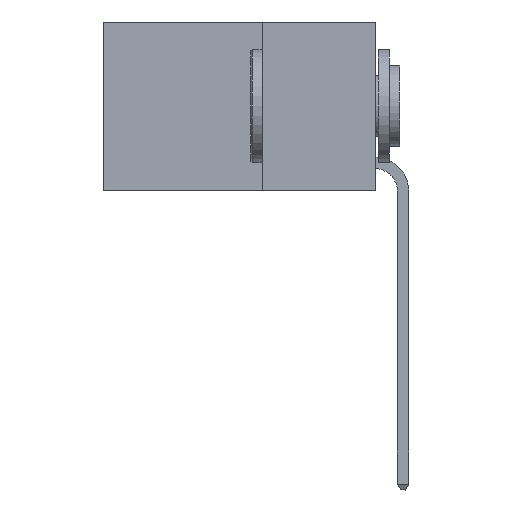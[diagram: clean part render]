
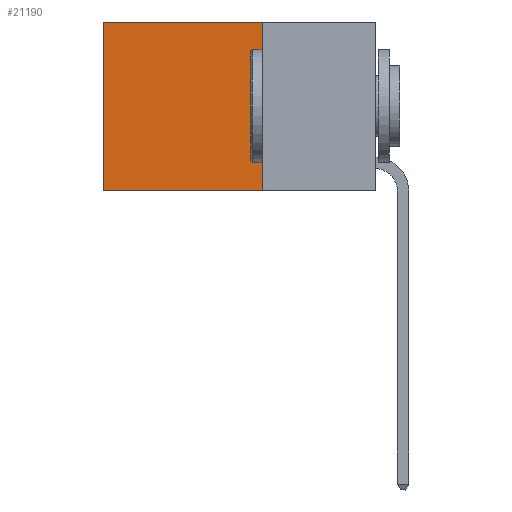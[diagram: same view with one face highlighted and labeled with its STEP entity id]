
A CAD part, left-side view. The second image highlights one B-rep face of the part: STEP entity #21190.
In plain terms, the highlighted planar face has unit normal (-1, 0, 0).
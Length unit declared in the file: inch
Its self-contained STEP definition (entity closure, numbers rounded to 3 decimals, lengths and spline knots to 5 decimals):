
#2144 = DIRECTION ( 'NONE',  ( 0., 1., 0. ) ) ;
#2157 = CARTESIAN_POINT ( 'NONE',  ( 0.2625, 0.25, 0. ) ) ;
#2172 = CARTESIAN_POINT ( 'NONE',  ( 0.2625, 0.6, 0. ) ) ;
#2182 = VECTOR ( 'NONE', #5967, 39.37008 ) ;
#2566 = CARTESIAN_POINT ( 'NONE',  ( 0.2625, 0.25, 0. ) ) ;
#3322 = VERTEX_POINT ( 'NONE', #19177 ) ;
#3429 = DIRECTION ( 'NONE',  ( 0., 0., -1. ) ) ;
#5967 = DIRECTION ( 'NONE',  ( 0., 1., 0. ) ) ;
#7459 = VERTEX_POINT ( 'NONE', #13827 ) ;
#7575 = CARTESIAN_POINT ( 'NONE',  ( 0.2625, 0.25, -0.37 ) ) ;
#7764 = ORIENTED_EDGE ( 'NONE', *, *, #11407, .T. ) ;
#7825 = LINE ( 'NONE', #2157, #2182 ) ;
#7829 = VECTOR ( 'NONE', #2144, 39.37008 ) ;
#9007 = EDGE_CURVE ( 'NONE', #7459, #3322, #13155, .T. ) ;
#11407 = EDGE_CURVE ( 'NONE', #19480, #3322, #18967, .T. ) ;
#11421 = LINE ( 'NONE', #16744, #15917 ) ;
#11435 = DIRECTION ( 'NONE',  ( 1., 0., 0. ) ) ;
#11440 = EDGE_LOOP ( 'NONE', ( #7764, #14529, #12044, #15341 ) ) ;
#11797 = EDGE_CURVE ( 'NONE', #14959, #19480, #7825, .T. ) ;
#12044 = ORIENTED_EDGE ( 'NONE', *, *, #20227, .F. ) ;
#13155 = LINE ( 'NONE', #7575, #7829 ) ;
#13446 = CARTESIAN_POINT ( 'NONE',  ( 0.2625, 0.25, 0. ) ) ;
#13447 = DIRECTION ( 'NONE',  ( 0., 0., -1. ) ) ;
#13827 = CARTESIAN_POINT ( 'NONE',  ( 0.2625, 0.25, -0.37 ) ) ;
#14010 = AXIS2_PLACEMENT_3D ( 'NONE', #2566, #11435, #22887 ) ;
#14529 = ORIENTED_EDGE ( 'NONE', *, *, #9007, .F. ) ;
#14959 = VERTEX_POINT ( 'NONE', #13446 ) ;
#15328 = PLANE ( 'NONE',  #14010 ) ;
#15341 = ORIENTED_EDGE ( 'NONE', *, *, #11797, .T. ) ;
#15696 = FACE_OUTER_BOUND ( 'NONE', #11440, .T. ) ;
#15917 = VECTOR ( 'NONE', #3429, 39.37008 ) ;
#16744 = CARTESIAN_POINT ( 'NONE',  ( 0.2625, 0.25, 0. ) ) ;
#18967 = LINE ( 'NONE', #22363, #23864 ) ;
#19177 = CARTESIAN_POINT ( 'NONE',  ( 0.2625, 0.6, -0.37 ) ) ;
#19480 = VERTEX_POINT ( 'NONE', #2172 ) ;
#20227 = EDGE_CURVE ( 'NONE', #14959, #7459, #11421, .T. ) ;
#21190 = ADVANCED_FACE ( 'NONE', ( #15696 ), #15328, .F. ) ;
#22363 = CARTESIAN_POINT ( 'NONE',  ( 0.2625, 0.6, 0. ) ) ;
#22887 = DIRECTION ( 'NONE',  ( 0., 0., -1. ) ) ;
#23864 = VECTOR ( 'NONE', #13447, 39.37008 ) ;
